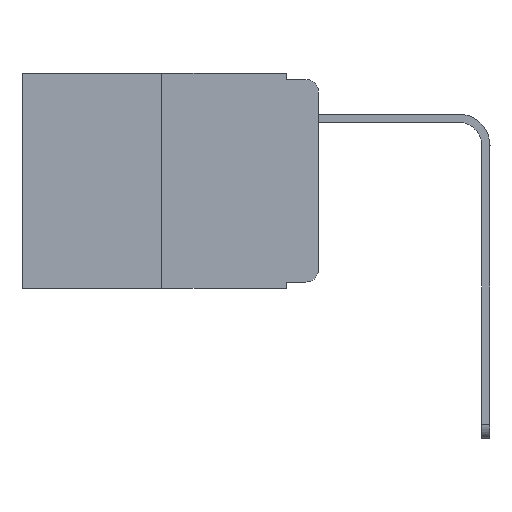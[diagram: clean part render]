
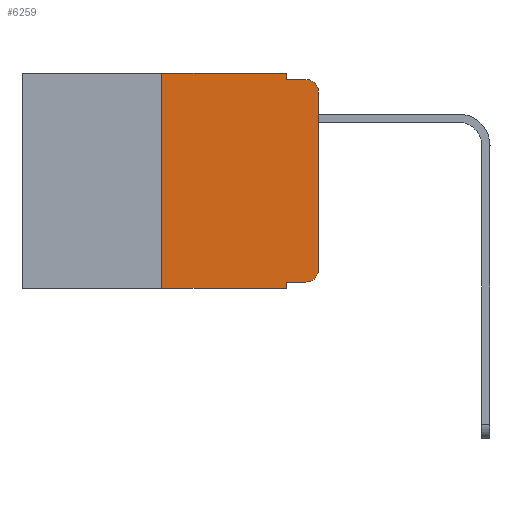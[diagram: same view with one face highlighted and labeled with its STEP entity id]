
A CAD part, left-side view. The second image highlights one B-rep face of the part: STEP entity #6259.
In plain terms, the highlighted planar face has unit normal (-1, 0, 0).
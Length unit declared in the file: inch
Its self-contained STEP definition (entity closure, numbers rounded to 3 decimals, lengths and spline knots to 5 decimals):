
#116 = CARTESIAN_POINT ( 'NONE',  ( 0., 0.051, 0. ) ) ;
#123 = CARTESIAN_POINT ( 'NONE',  ( 0., 0.473, 0. ) ) ;
#376 = ORIENTED_EDGE ( 'NONE', *, *, #8488, .T. ) ;
#438 = CARTESIAN_POINT ( 'NONE',  ( 0., 0.02, -0.01 ) ) ;
#453 = EDGE_CURVE ( 'NONE', #2495, #3759, #3715, .T. ) ;
#507 = EDGE_CURVE ( 'NONE', #566, #3321, #11177, .T. ) ;
#566 = VERTEX_POINT ( 'NONE', #7660 ) ;
#629 = CARTESIAN_POINT ( 'NONE',  ( 0., 0.051, -0.333 ) ) ;
#801 = CARTESIAN_POINT ( 'NONE',  ( 0., 0.02, -0.313 ) ) ;
#1064 = LINE ( 'NONE', #12814, #8774 ) ;
#1205 = DIRECTION ( 'NONE',  ( 0., -1., 0. ) ) ;
#1298 = VECTOR ( 'NONE', #9267, 39.37008 ) ;
#1325 = CIRCLE ( 'NONE', #12770, 0.02 ) ;
#1383 = EDGE_LOOP ( 'NONE', ( #6674, #3501, #12445, #7450, #11967, #9731, #376, #7035, #11583, #8942 ) ) ;
#1456 = CARTESIAN_POINT ( 'NONE',  ( 0., 0.25, 0. ) ) ;
#1586 = DIRECTION ( 'NONE',  ( 0., -1., 0. ) ) ;
#1722 = DIRECTION ( 'NONE',  ( 0., -1., 0. ) ) ;
#1762 = EDGE_CURVE ( 'NONE', #13277, #6581, #9353, .T. ) ;
#1785 = DIRECTION ( 'NONE',  ( 0., 0., -1. ) ) ;
#2495 = VERTEX_POINT ( 'NONE', #629 ) ;
#2673 = VECTOR ( 'NONE', #1722, 39.37008 ) ;
#3321 = VERTEX_POINT ( 'NONE', #5051 ) ;
#3501 = ORIENTED_EDGE ( 'NONE', *, *, #4132, .T. ) ;
#3524 = VECTOR ( 'NONE', #1205, 39.37008 ) ;
#3715 = LINE ( 'NONE', #116, #6970 ) ;
#3750 = DIRECTION ( 'NONE',  ( 0., 0., -1. ) ) ;
#3759 = VERTEX_POINT ( 'NONE', #10097 ) ;
#3870 = LINE ( 'NONE', #13160, #7907 ) ;
#3987 = CARTESIAN_POINT ( 'NONE',  ( 0., 0.051, -0.333 ) ) ;
#4132 = EDGE_CURVE ( 'NONE', #6581, #5928, #5808, .T. ) ;
#4781 = CARTESIAN_POINT ( 'NONE',  ( 0., 0.473, 0. ) ) ;
#4983 = VECTOR ( 'NONE', #6518, 39.37008 ) ;
#5051 = CARTESIAN_POINT ( 'NONE',  ( 0., 0.25, 0. ) ) ;
#5658 = EDGE_CURVE ( 'NONE', #2495, #7846, #9498, .T. ) ;
#5808 = CIRCLE ( 'NONE', #6081, 0.02 ) ;
#5928 = VERTEX_POINT ( 'NONE', #438 ) ;
#5947 = CARTESIAN_POINT ( 'NONE',  ( 0., 0., -0.03 ) ) ;
#5971 = DIRECTION ( 'NONE',  ( -1., 0., 0. ) ) ;
#6081 = AXIS2_PLACEMENT_3D ( 'NONE', #7942, #5971, #1785 ) ;
#6259 = ADVANCED_FACE ( 'NONE', ( #12569 ), #9017, .F. ) ;
#6518 = DIRECTION ( 'NONE',  ( 0., 0., 1. ) ) ;
#6581 = VERTEX_POINT ( 'NONE', #5947 ) ;
#6674 = ORIENTED_EDGE ( 'NONE', *, *, #1762, .T. ) ;
#6947 = DIRECTION ( 'NONE',  ( 0., 0., -1. ) ) ;
#6970 = VECTOR ( 'NONE', #7663, 39.37008 ) ;
#7035 = ORIENTED_EDGE ( 'NONE', *, *, #453, .F. ) ;
#7450 = ORIENTED_EDGE ( 'NONE', *, *, #9037, .F. ) ;
#7660 = CARTESIAN_POINT ( 'NONE',  ( 0., 0.25, -0.343 ) ) ;
#7663 = DIRECTION ( 'NONE',  ( 0., 0., -1. ) ) ;
#7846 = VERTEX_POINT ( 'NONE', #8247 ) ;
#7907 = VECTOR ( 'NONE', #11000, 39.37008 ) ;
#7921 = DIRECTION ( 'NONE',  ( 1., 0., 0. ) ) ;
#7942 = CARTESIAN_POINT ( 'NONE',  ( 0., 0.02, -0.03 ) ) ;
#7994 = DIRECTION ( 'NONE',  ( -1., 0., 0. ) ) ;
#8247 = CARTESIAN_POINT ( 'NONE',  ( 0., 0.02, -0.333 ) ) ;
#8477 = LINE ( 'NONE', #13047, #2673 ) ;
#8488 = EDGE_CURVE ( 'NONE', #566, #3759, #8477, .T. ) ;
#8774 = VECTOR ( 'NONE', #1586, 39.37008 ) ;
#8942 = ORIENTED_EDGE ( 'NONE', *, *, #9027, .T. ) ;
#9017 = PLANE ( 'NONE',  #9810 ) ;
#9027 = EDGE_CURVE ( 'NONE', #7846, #13277, #1325, .T. ) ;
#9037 = EDGE_CURVE ( 'NONE', #12499, #11961, #3870, .T. ) ;
#9267 = DIRECTION ( 'NONE',  ( 0., -1., 0. ) ) ;
#9353 = LINE ( 'NONE', #10642, #4983 ) ;
#9498 = LINE ( 'NONE', #3987, #1298 ) ;
#9731 = ORIENTED_EDGE ( 'NONE', *, *, #507, .F. ) ;
#9810 = AXIS2_PLACEMENT_3D ( 'NONE', #4781, #7921, #6947 ) ;
#10097 = CARTESIAN_POINT ( 'NONE',  ( 0., 0.051, -0.343 ) ) ;
#10250 = CARTESIAN_POINT ( 'NONE',  ( 0., 0., -0.313 ) ) ;
#10455 = EDGE_CURVE ( 'NONE', #3321, #12499, #11923, .T. ) ;
#10642 = CARTESIAN_POINT ( 'NONE',  ( 0., 0., 0. ) ) ;
#10818 = CARTESIAN_POINT ( 'NONE',  ( 0., 0.051, -0.01 ) ) ;
#10854 = VECTOR ( 'NONE', #11939, 39.37008 ) ;
#11000 = DIRECTION ( 'NONE',  ( 0., 0., -1. ) ) ;
#11177 = LINE ( 'NONE', #1456, #10854 ) ;
#11583 = ORIENTED_EDGE ( 'NONE', *, *, #5658, .T. ) ;
#11923 = LINE ( 'NONE', #123, #3524 ) ;
#11939 = DIRECTION ( 'NONE',  ( 0., 0., 1. ) ) ;
#11961 = VERTEX_POINT ( 'NONE', #10818 ) ;
#11967 = ORIENTED_EDGE ( 'NONE', *, *, #10455, .F. ) ;
#12445 = ORIENTED_EDGE ( 'NONE', *, *, #13311, .F. ) ;
#12499 = VERTEX_POINT ( 'NONE', #12573 ) ;
#12569 = FACE_OUTER_BOUND ( 'NONE', #1383, .T. ) ;
#12573 = CARTESIAN_POINT ( 'NONE',  ( 0., 0.051, 0. ) ) ;
#12770 = AXIS2_PLACEMENT_3D ( 'NONE', #801, #7994, #3750 ) ;
#12814 = CARTESIAN_POINT ( 'NONE',  ( 0., 0.051, -0.01 ) ) ;
#13047 = CARTESIAN_POINT ( 'NONE',  ( 0., 0.473, -0.343 ) ) ;
#13160 = CARTESIAN_POINT ( 'NONE',  ( 0., 0.051, 0. ) ) ;
#13277 = VERTEX_POINT ( 'NONE', #10250 ) ;
#13311 = EDGE_CURVE ( 'NONE', #11961, #5928, #1064, .T. ) ;
